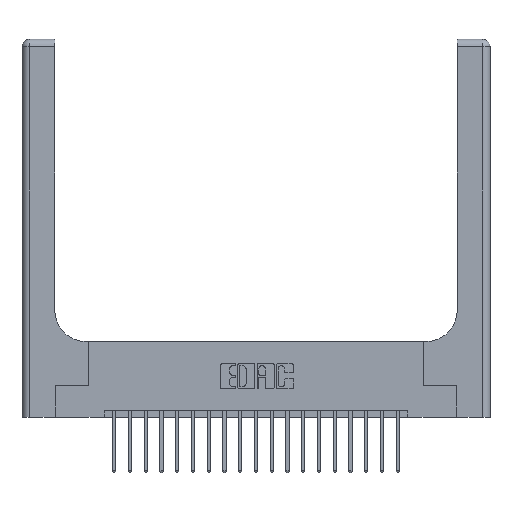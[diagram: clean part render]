
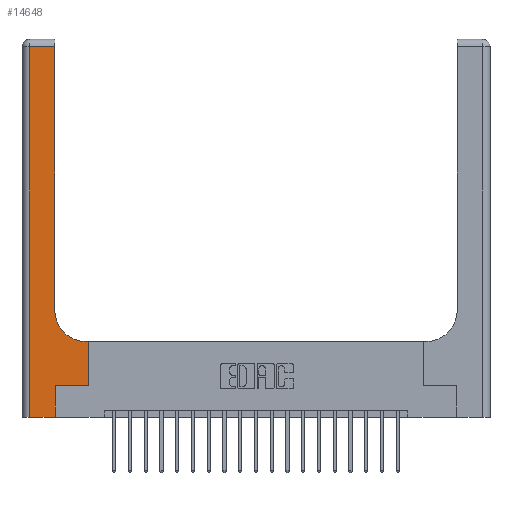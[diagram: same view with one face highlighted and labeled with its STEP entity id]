
A CAD part, top view. The second image highlights one B-rep face of the part: STEP entity #14648.
In plain terms, the highlighted planar face has unit normal (0, 0, 1).
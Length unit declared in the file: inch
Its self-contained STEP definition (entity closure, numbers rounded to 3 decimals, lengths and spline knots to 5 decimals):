
#4 = CARTESIAN_POINT ( 'NONE',  ( 0.06, 0., 0.37 ) ) ;
#629 = CARTESIAN_POINT ( 'NONE',  ( 0.26, 0.6, 0.37 ) ) ;
#768 = VERTEX_POINT ( 'NONE', #5521 ) ;
#931 = LINE ( 'NONE', #7798, #20637 ) ;
#1291 = DIRECTION ( 'NONE',  ( 0., 1., 0. ) ) ;
#1551 = CARTESIAN_POINT ( 'NONE',  ( 0.265, 0.25, 0.37 ) ) ;
#2492 = AXIS2_PLACEMENT_3D ( 'NONE', #15936, #6194, #9818 ) ;
#2918 = ORIENTED_EDGE ( 'NONE', *, *, #8591, .T. ) ;
#3216 = CARTESIAN_POINT ( 'NONE',  ( 0.265, 0., 0.37 ) ) ;
#3493 = DIRECTION ( 'NONE',  ( 0., 0., -1. ) ) ;
#3780 = DIRECTION ( 'NONE',  ( 0., 1., 0. ) ) ;
#3809 = EDGE_CURVE ( 'NONE', #14695, #768, #9443, .T. ) ;
#4081 = DIRECTION ( 'NONE',  ( 0., -1., 0. ) ) ;
#4127 = ORIENTED_EDGE ( 'NONE', *, *, #18859, .T. ) ;
#4227 = EDGE_CURVE ( 'NONE', #13796, #18906, #11738, .T. ) ;
#4386 = LINE ( 'NONE', #1551, #14988 ) ;
#5136 = CARTESIAN_POINT ( 'NONE',  ( 0.265, 0., 0.37 ) ) ;
#5521 = CARTESIAN_POINT ( 'NONE',  ( 0.528, 0.6, 0.37 ) ) ;
#5784 = VERTEX_POINT ( 'NONE', #17832 ) ;
#5927 = VECTOR ( 'NONE', #21100, 39.37008 ) ;
#6049 = CARTESIAN_POINT ( 'NONE',  ( 0., 0., 0.37 ) ) ;
#6194 = DIRECTION ( 'NONE',  ( 0., 0., -1. ) ) ;
#6966 = VECTOR ( 'NONE', #20226, 39.37008 ) ;
#7090 = CARTESIAN_POINT ( 'NONE',  ( 0., 3., 0.37 ) ) ;
#7798 = CARTESIAN_POINT ( 'NONE',  ( 0.06, 3., 0.37 ) ) ;
#8591 = EDGE_CURVE ( 'NONE', #16122, #14695, #4386, .T. ) ;
#8742 = LINE ( 'NONE', #5136, #9319 ) ;
#9319 = VECTOR ( 'NONE', #19976, 39.37008 ) ;
#9356 = LINE ( 'NONE', #6049, #5927 ) ;
#9443 = LINE ( 'NONE', #15985, #15481 ) ;
#9518 = CARTESIAN_POINT ( 'NONE',  ( 0.26, 2.94, 0.37 ) ) ;
#9818 = DIRECTION ( 'NONE',  ( 1., 0., 0. ) ) ;
#9974 = EDGE_CURVE ( 'NONE', #14069, #5784, #13043, .T. ) ;
#10094 = FACE_OUTER_BOUND ( 'NONE', #12075, .T. ) ;
#10157 = ORIENTED_EDGE ( 'NONE', *, *, #15040, .T. ) ;
#10174 = LINE ( 'NONE', #13183, #15360 ) ;
#10431 = ORIENTED_EDGE ( 'NONE', *, *, #3809, .T. ) ;
#11738 = CIRCLE ( 'NONE', #2492, 0.25 ) ;
#11996 = VECTOR ( 'NONE', #12842, 39.37008 ) ;
#12075 = EDGE_LOOP ( 'NONE', ( #10157, #18898, #4127, #20638, #20562, #2918, #10431, #15768, #13002 ) ) ;
#12426 = EDGE_CURVE ( 'NONE', #768, #13796, #15338, .T. ) ;
#12842 = DIRECTION ( 'NONE',  ( -1., 0., 0. ) ) ;
#13002 = ORIENTED_EDGE ( 'NONE', *, *, #4227, .T. ) ;
#13043 = LINE ( 'NONE', #19531, #11996 ) ;
#13183 = CARTESIAN_POINT ( 'NONE',  ( 0.26, 3., 0.37 ) ) ;
#13796 = VERTEX_POINT ( 'NONE', #19988 ) ;
#14069 = VERTEX_POINT ( 'NONE', #9518 ) ;
#14648 = ADVANCED_FACE ( 'NONE', ( #10094 ), #18236, .F. ) ;
#14695 = VERTEX_POINT ( 'NONE', #15146 ) ;
#14838 = VERTEX_POINT ( 'NONE', #4 ) ;
#14988 = VECTOR ( 'NONE', #16034, 39.37008 ) ;
#15040 = EDGE_CURVE ( 'NONE', #18906, #14069, #10174, .T. ) ;
#15146 = CARTESIAN_POINT ( 'NONE',  ( 0.528, 0.25, 0.37 ) ) ;
#15309 = VERTEX_POINT ( 'NONE', #3216 ) ;
#15338 = LINE ( 'NONE', #629, #6966 ) ;
#15360 = VECTOR ( 'NONE', #3780, 39.37008 ) ;
#15481 = VECTOR ( 'NONE', #1291, 39.37008 ) ;
#15768 = ORIENTED_EDGE ( 'NONE', *, *, #12426, .T. ) ;
#15936 = CARTESIAN_POINT ( 'NONE',  ( 0.51, 0.85, 0.37 ) ) ;
#15985 = CARTESIAN_POINT ( 'NONE',  ( 0.528, 0.25, 0.37 ) ) ;
#16034 = DIRECTION ( 'NONE',  ( 1., 0., 0. ) ) ;
#16122 = VERTEX_POINT ( 'NONE', #17966 ) ;
#16300 = EDGE_CURVE ( 'NONE', #15309, #16122, #8742, .T. ) ;
#17832 = CARTESIAN_POINT ( 'NONE',  ( 0.06, 2.94, 0.37 ) ) ;
#17966 = CARTESIAN_POINT ( 'NONE',  ( 0.265, 0.25, 0.37 ) ) ;
#18236 = PLANE ( 'NONE',  #19697 ) ;
#18641 = EDGE_CURVE ( 'NONE', #14838, #15309, #9356, .T. ) ;
#18859 = EDGE_CURVE ( 'NONE', #5784, #14838, #931, .T. ) ;
#18898 = ORIENTED_EDGE ( 'NONE', *, *, #9974, .T. ) ;
#18906 = VERTEX_POINT ( 'NONE', #20298 ) ;
#19531 = CARTESIAN_POINT ( 'NONE',  ( 0., 2.94, 0.37 ) ) ;
#19697 = AXIS2_PLACEMENT_3D ( 'NONE', #7090, #3493, #19915 ) ;
#19915 = DIRECTION ( 'NONE',  ( -1., 0., 0. ) ) ;
#19976 = DIRECTION ( 'NONE',  ( 0., 1., 0. ) ) ;
#19988 = CARTESIAN_POINT ( 'NONE',  ( 0.51, 0.6, 0.37 ) ) ;
#20226 = DIRECTION ( 'NONE',  ( -1., 0., 0. ) ) ;
#20298 = CARTESIAN_POINT ( 'NONE',  ( 0.26, 0.85, 0.37 ) ) ;
#20562 = ORIENTED_EDGE ( 'NONE', *, *, #16300, .T. ) ;
#20637 = VECTOR ( 'NONE', #4081, 39.37008 ) ;
#20638 = ORIENTED_EDGE ( 'NONE', *, *, #18641, .T. ) ;
#21100 = DIRECTION ( 'NONE',  ( 1., 0., 0. ) ) ;
